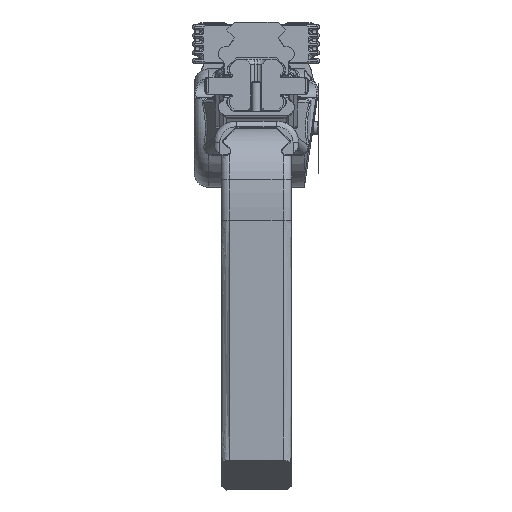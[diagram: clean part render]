
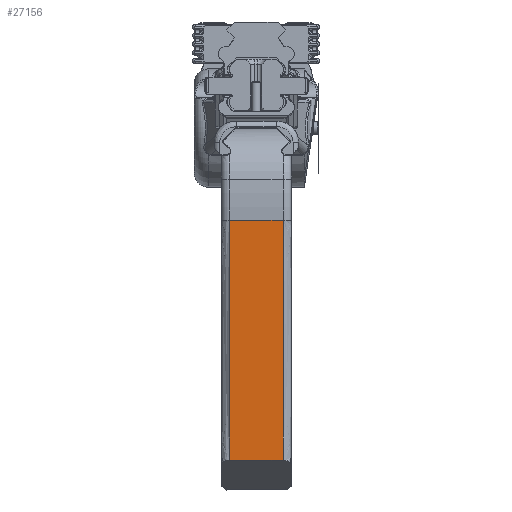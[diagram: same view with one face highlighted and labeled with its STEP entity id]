
A CAD part, left-side view. The second image highlights one B-rep face of the part: STEP entity #27156.
In plain terms, the highlighted free-form (B-spline) face has degree [1, 2] with [2, 3] control points.
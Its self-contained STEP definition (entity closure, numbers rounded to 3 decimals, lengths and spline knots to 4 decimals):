
#470=(
BOUNDED_SURFACE()
B_SPLINE_SURFACE(1,2,((#48382,#48383,#48384),(#48385,#48386,#48387)),
 .UNSPECIFIED.,.F.,.F.,.F.)
B_SPLINE_SURFACE_WITH_KNOTS((2,2),(3,3),(0.022,0.033),
(-0.0715,-0.0043),.UNSPECIFIED.)
GEOMETRIC_REPRESENTATION_ITEM()
RATIONAL_B_SPLINE_SURFACE(((1.,0.999,1.),(1.,0.999,
1.)))
REPRESENTATION_ITEM($)
SURFACE()
);
#1594=B_SPLINE_CURVE_WITH_KNOTS($,3,(#48377,#48378,#48379,#48380),
 .UNSPECIFIED.,.F.,.F.,(4,4),(2.1307,10.6591),
 .UNSPECIFIED.);
#1595=B_SPLINE_CURVE_WITH_KNOTS($,3,(#48389,#48390,#48391,#48392),
 .UNSPECIFIED.,.F.,.F.,(4,4),(0.,8.5284),.UNSPECIFIED.);
#3006=FACE_OUTER_BOUND($,#4889,.T.);
#4889=EDGE_LOOP($,(#21323,#21324,#21325,#21326));
#8527=LINE($,#48089,#10269);
#8555=LINE($,#48393,#10297);
#10269=VECTOR($,#35055,1.8974);
#10297=VECTOR($,#35101,1.8974);
#12337=VERTEX_POINT($,#48075);
#12338=VERTEX_POINT($,#48088);
#12364=VERTEX_POINT($,#48376);
#12365=VERTEX_POINT($,#48388);
#15517=EDGE_CURVE($,#12338,#12337,#8527,.T.);
#15559=EDGE_CURVE($,#12338,#12364,#1594,.T.);
#15561=EDGE_CURVE($,#12365,#12337,#1595,.T.);
#15562=EDGE_CURVE($,#12364,#12365,#8555,.T.);
#21323=ORIENTED_EDGE($,*,*,#15517,.T.);
#21324=ORIENTED_EDGE($,*,*,#15561,.F.);
#21325=ORIENTED_EDGE($,*,*,#15562,.F.);
#21326=ORIENTED_EDGE($,*,*,#15559,.F.);
#27156=ADVANCED_FACE($,(#3006),#470,.T.);
#35055=DIRECTION($,(0.,-1.,0.));
#35101=DIRECTION($,(0.,-1.,0.));
#48075=CARTESIAN_POINT('',(-32.2256,-0.9487,3.2427));
#48088=CARTESIAN_POINT('',(-32.2256,0.9487,3.2427));
#48089=CARTESIAN_POINT($,(-32.2256,0.,3.2427));
#48376=CARTESIAN_POINT('',(-32.6645,0.9487,11.7294));
#48377=CARTESIAN_POINT('Ctrl Pts',(-32.2256,0.9487,
3.2427));
#48378=CARTESIAN_POINT('Ctrl Pts',(-32.2424,0.9487,
6.0763));
#48379=CARTESIAN_POINT('Ctrl Pts',(-32.3892,0.9487,
8.9091));
#48380=CARTESIAN_POINT('Ctrl Pts',(-32.6645,0.9487,
11.7294));
#48382=CARTESIAN_POINT('Ctrl Pts',(-32.6645,-0.9487,
11.7294));
#48383=CARTESIAN_POINT('Ctrl Pts',(-32.2507,-0.9487,
7.4915));
#48384=CARTESIAN_POINT('Ctrl Pts',(-32.2256,-0.9487,
3.2427));
#48385=CARTESIAN_POINT('Ctrl Pts',(-32.6645,0.9487,11.7294));
#48386=CARTESIAN_POINT('Ctrl Pts',(-32.2507,0.9487,
7.4915));
#48387=CARTESIAN_POINT('Ctrl Pts',(-32.2256,0.9487,
3.2427));
#48388=CARTESIAN_POINT('',(-32.6645,-0.9487,11.7294));
#48389=CARTESIAN_POINT('Ctrl Pts',(-32.6645,-0.9487,
11.7294));
#48390=CARTESIAN_POINT('Ctrl Pts',(-32.3892,-0.9487,
8.9091));
#48391=CARTESIAN_POINT('Ctrl Pts',(-32.2424,-0.9487,6.0763));
#48392=CARTESIAN_POINT('Ctrl Pts',(-32.2256,-0.9487,
3.2427));
#48393=CARTESIAN_POINT($,(-32.6645,-2.3744,11.7294));
